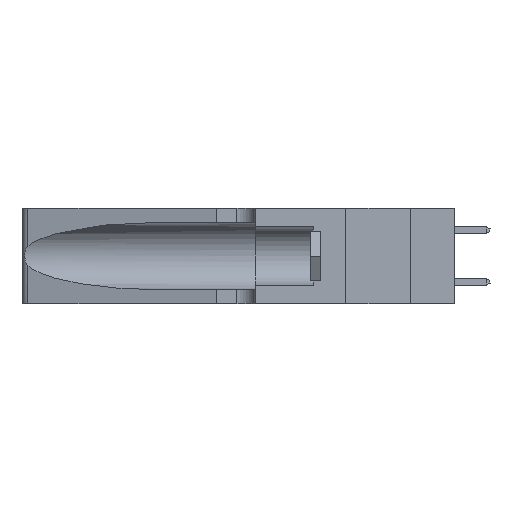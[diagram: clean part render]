
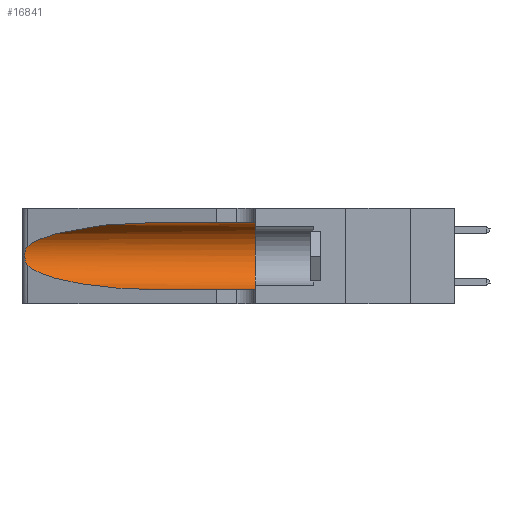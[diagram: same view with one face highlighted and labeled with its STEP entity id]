
A CAD part, left-side view. The second image highlights one B-rep face of the part: STEP entity #16841.
In plain terms, the highlighted cylindrical face has radius 3.308 mm (diameter 6.617 mm), a partial arc.
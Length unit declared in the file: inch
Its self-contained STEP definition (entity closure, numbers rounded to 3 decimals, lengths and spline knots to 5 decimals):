
#248 = ORIENTED_EDGE ( 'NONE', *, *, #12288, .T. ) ;
#417 = CARTESIAN_POINT ( 'NONE',  ( 0.25487, 1.22718, 0.14631 ) ) ;
#437 = VERTEX_POINT ( 'NONE', #417 ) ;
#448 = CARTESIAN_POINT ( 'NONE',  ( 0.1305, 0.72297, 0.31525 ) ) ;
#1607 = CYLINDRICAL_SURFACE ( 'NONE', #23654, 0.13025 ) ;
#2264 = CARTESIAN_POINT ( 'NONE',  ( 0.25487, 1.22718, 0.22369 ) ) ;
#2384 = CARTESIAN_POINT ( 'NONE',  ( 0.25639, 1.23186, 0.15144 ) ) ;
#2611 = DIRECTION ( 'NONE',  ( 0., -1., 0. ) ) ;
#2942 = AXIS2_PLACEMENT_3D ( 'NONE', #23823, #7426, #26512 ) ;
#4588 = VERTEX_POINT ( 'NONE', #32895 ) ;
#4830 = DIRECTION ( 'NONE',  ( 0., 0., -1. ) ) ;
#4957 = B_SPLINE_CURVE_WITH_KNOTS ( 'NONE', 3,
 ( #2264, #13231, #7844, #26903, #10603, #29551, #13351, #32245, #16144, #34919, #18892, #2384, #21623, #5157 ),
 .UNSPECIFIED., .F., .F.,
 ( 4, 2, 2, 2, 2, 2, 4 ),
 ( 0., 0.00027, 0.00053, 0.00107, 0.0016, 0.00187, 0.00214 ),
 .UNSPECIFIED. ) ;
#5157 = CARTESIAN_POINT ( 'NONE',  ( 0.25487, 1.22718, 0.14631 ) ) ;
#7426 = DIRECTION ( 'NONE',  ( 0., 1., 0. ) ) ;
#7676 = VERTEX_POINT ( 'NONE', #19817 ) ;
#7844 = CARTESIAN_POINT ( 'NONE',  ( 0.25639, 1.23184, 0.21858 ) ) ;
#8410 = CARTESIAN_POINT ( 'NONE',  ( 0.25487, 1.22718, 0.22369 ) ) ;
#8734 = ORIENTED_EDGE ( 'NONE', *, *, #30314, .T. ) ;
#8834 = CARTESIAN_POINT ( 'NONE',  ( 0.25487, 1.22718, 0.22369 ) ) ;
#9924 = CIRCLE ( 'NONE', #2942, 0.13025 ) ;
#10603 = CARTESIAN_POINT ( 'NONE',  ( 0.25854, 1.2359, 0.20912 ) ) ;
#11921 = ORIENTED_EDGE ( 'NONE', *, *, #33177, .T. ) ;
#12254 = CARTESIAN_POINT ( 'NONE',  ( 0.2373, 1.15595, 0.08982 ) ) ;
#12288 = EDGE_CURVE ( 'NONE', #24777, #437, #4957, .T. ) ;
#13231 = CARTESIAN_POINT ( 'NONE',  ( 0.25555, 1.22994, 0.2215 ) ) ;
#13351 = CARTESIAN_POINT ( 'NONE',  ( 0.26075, 1.23896, 0.19203 ) ) ;
#13439 = VECTOR ( 'NONE', #2611, 39.37008 ) ;
#13807 = EDGE_CURVE ( 'NONE', #14689, #24777, #33912, .T. ) ;
#13977 = EDGE_LOOP ( 'NONE', ( #21744, #248, #8734, #11921, #30842, #25877 ) ) ;
#14689 = VERTEX_POINT ( 'NONE', #20380 ) ;
#15813 = DIRECTION ( 'NONE',  ( 0., -1., 0. ) ) ;
#16135 = EDGE_CURVE ( 'NONE', #22557, #4588, #9924, .T. ) ;
#16144 = CARTESIAN_POINT ( 'NONE',  ( 0.26017, 1.23833, 0.17102 ) ) ;
#16309 = FACE_OUTER_BOUND ( 'NONE', #13977, .T. ) ;
#16403 = CARTESIAN_POINT ( 'NONE',  ( 0.1305, 1.61858, 0.31525 ) ) ;
#16841 = ADVANCED_FACE ( 'NONE', ( #16309 ), #1607, .F. ) ;
#17034 = CARTESIAN_POINT ( 'NONE',  ( 0.18966, 0.96281, 0.31525 ) ) ;
#17808 = CARTESIAN_POINT ( 'NONE',  ( 0.1305, 0.72297, 0.05475 ) ) ;
#18892 = CARTESIAN_POINT ( 'NONE',  ( 0.25789, 1.23486, 0.15765 ) ) ;
#19817 = CARTESIAN_POINT ( 'NONE',  ( 0.1305, 0.72297, 0.05475 ) ) ;
#20380 = CARTESIAN_POINT ( 'NONE',  ( 0.1305, 0.72297, 0.31525 ) ) ;
#20405 = LINE ( 'NONE', #16403, #26697 ) ;
#20846 = CARTESIAN_POINT ( 'NONE',  ( 0.1305, 0.35, 0.31525 ) ) ;
#21286 = CARTESIAN_POINT ( 'NONE',  ( 0.1305, 1.61858, 0.185 ) ) ;
#21588 = LINE ( 'NONE', #24649, #13439 ) ;
#21623 = CARTESIAN_POINT ( 'NONE',  ( 0.25555, 1.22993, 0.14849 ) ) ;
#21744 = ORIENTED_EDGE ( 'NONE', *, *, #13807, .T. ) ;
#22557 = VERTEX_POINT ( 'NONE', #20846 ) ;
#23654 = AXIS2_PLACEMENT_3D ( 'NONE', #21286, #15813, #4830 ) ;
#23823 = CARTESIAN_POINT ( 'NONE',  ( 0.1305, 0.35, 0.185 ) ) ;
#24649 = CARTESIAN_POINT ( 'NONE',  ( 0.1305, 1.61858, 0.05475 ) ) ;
#24777 = VERTEX_POINT ( 'NONE', #8410 ) ;
#25172 = CARTESIAN_POINT ( 'NONE',  ( 0.2373, 1.15595, 0.28018 ) ) ;
#25843 = CARTESIAN_POINT ( 'NONE',  ( 0.25487, 1.22718, 0.14631 ) ) ;
#25877 = ORIENTED_EDGE ( 'NONE', *, *, #26078, .F. ) ;
#26078 = EDGE_CURVE ( 'NONE', #14689, #22557, #20405, .T. ) ;
#26512 = DIRECTION ( 'NONE',  ( 0., 0., 1. ) ) ;
#26697 = VECTOR ( 'NONE', #35168, 39.37008 ) ;
#26903 = CARTESIAN_POINT ( 'NONE',  ( 0.25787, 1.23484, 0.2124 ) ) ;
#29551 = CARTESIAN_POINT ( 'NONE',  ( 0.26018, 1.23835, 0.19895 ) ) ;
#30314 = EDGE_CURVE ( 'NONE', #437, #7676, #31331, .T. ) ;
#30842 = ORIENTED_EDGE ( 'NONE', *, *, #16135, .F. ) ;
#31331 =( BOUNDED_CURVE ( )  B_SPLINE_CURVE ( 3, ( #25843, #12254, #33868, #17808 ),
 .UNSPECIFIED., .F., .F. ) 
 B_SPLINE_CURVE_WITH_KNOTS ( ( 4, 4 ),
 ( 3.44316, 4.71239 ),
 .UNSPECIFIED. ) 
 CURVE ( )  GEOMETRIC_REPRESENTATION_ITEM ( )  RATIONAL_B_SPLINE_CURVE ( ( 1., 0.87, 0.87, 1. ) ) 
 REPRESENTATION_ITEM ( '' )  );
#32245 = CARTESIAN_POINT ( 'NONE',  ( 0.26075, 1.23896, 0.178 ) ) ;
#32895 = CARTESIAN_POINT ( 'NONE',  ( 0.1305, 0.35, 0.05475 ) ) ;
#33177 = EDGE_CURVE ( 'NONE', #7676, #4588, #21588, .T. ) ;
#33868 = CARTESIAN_POINT ( 'NONE',  ( 0.18966, 0.96281, 0.05475 ) ) ;
#33912 =( BOUNDED_CURVE ( )  B_SPLINE_CURVE ( 3, ( #448, #17034, #25172, #8834 ),
 .UNSPECIFIED., .F., .F. ) 
 B_SPLINE_CURVE_WITH_KNOTS ( ( 4, 4 ),
 ( 1.5708, 2.84003 ),
 .UNSPECIFIED. ) 
 CURVE ( )  GEOMETRIC_REPRESENTATION_ITEM ( )  RATIONAL_B_SPLINE_CURVE ( ( 1., 0.87, 0.87, 1. ) ) 
 REPRESENTATION_ITEM ( '' )  );
#34919 = CARTESIAN_POINT ( 'NONE',  ( 0.25856, 1.23593, 0.16098 ) ) ;
#35168 = DIRECTION ( 'NONE',  ( 0., -1., 0. ) ) ;
